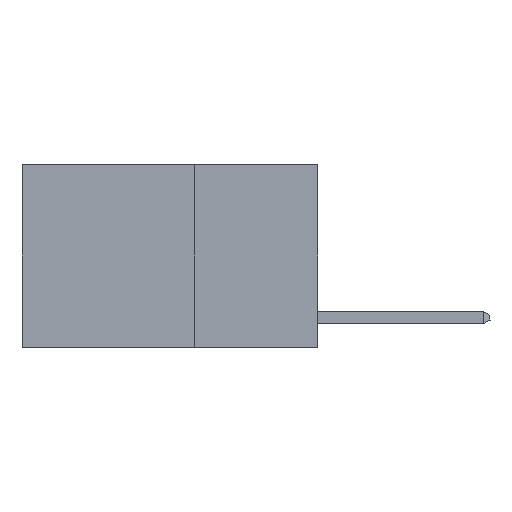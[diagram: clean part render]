
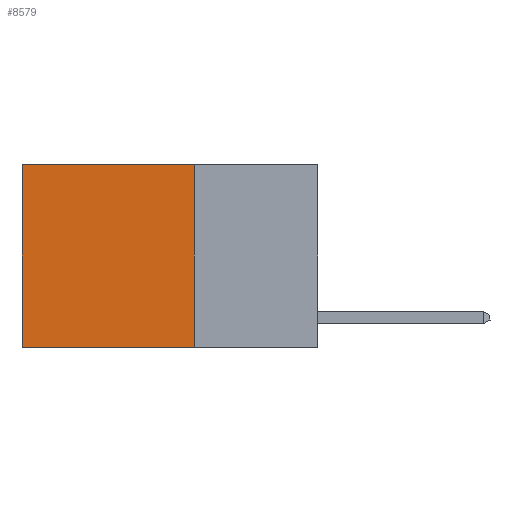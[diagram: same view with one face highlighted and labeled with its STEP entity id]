
A CAD part, left-side view. The second image highlights one B-rep face of the part: STEP entity #8579.
In plain terms, the highlighted planar face has unit normal (-1, 0, 0).
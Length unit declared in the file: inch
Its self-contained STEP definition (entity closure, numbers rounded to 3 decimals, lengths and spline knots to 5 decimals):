
#145 = CARTESIAN_POINT ( 'NONE',  ( 0.2625, 0.25, 0. ) ) ;
#263 = CARTESIAN_POINT ( 'NONE',  ( 0.2625, 0.6, -0.37 ) ) ;
#315 = ORIENTED_EDGE ( 'NONE', *, *, #9654, .F. ) ;
#1732 = VECTOR ( 'NONE', #3383, 39.37008 ) ;
#1985 = VERTEX_POINT ( 'NONE', #4915 ) ;
#2575 = VECTOR ( 'NONE', #4022, 39.37008 ) ;
#3164 = CARTESIAN_POINT ( 'NONE',  ( 0.2625, 0.25, -0.37 ) ) ;
#3243 = CARTESIAN_POINT ( 'NONE',  ( 0.2625, 0.25, 0. ) ) ;
#3383 = DIRECTION ( 'NONE',  ( 0., 0., -1. ) ) ;
#3748 = EDGE_CURVE ( 'NONE', #3813, #4988, #8011, .T. ) ;
#3813 = VERTEX_POINT ( 'NONE', #10590 ) ;
#4022 = DIRECTION ( 'NONE',  ( 0., 0., -1. ) ) ;
#4136 = ORIENTED_EDGE ( 'NONE', *, *, #3748, .T. ) ;
#4202 = FACE_OUTER_BOUND ( 'NONE', #13808, .T. ) ;
#4405 = DIRECTION ( 'NONE',  ( 0., 0., -1. ) ) ;
#4915 = CARTESIAN_POINT ( 'NONE',  ( 0.2625, 0.25, 0. ) ) ;
#4988 = VERTEX_POINT ( 'NONE', #263 ) ;
#5365 = EDGE_CURVE ( 'NONE', #7606, #4988, #7388, .T. ) ;
#7388 = LINE ( 'NONE', #3164, #13209 ) ;
#7606 = VERTEX_POINT ( 'NONE', #14103 ) ;
#7917 = DIRECTION ( 'NONE',  ( 0., 1., 0. ) ) ;
#8011 = LINE ( 'NONE', #15062, #1732 ) ;
#8446 = ORIENTED_EDGE ( 'NONE', *, *, #11267, .T. ) ;
#8579 = ADVANCED_FACE ( 'NONE', ( #4202 ), #10300, .F. ) ;
#9528 = LINE ( 'NONE', #145, #12562 ) ;
#9571 = DIRECTION ( 'NONE',  ( 0., 1., 0. ) ) ;
#9654 = EDGE_CURVE ( 'NONE', #1985, #7606, #11912, .T. ) ;
#10300 = PLANE ( 'NONE',  #13933 ) ;
#10590 = CARTESIAN_POINT ( 'NONE',  ( 0.2625, 0.6, 0. ) ) ;
#11267 = EDGE_CURVE ( 'NONE', #1985, #3813, #9528, .T. ) ;
#11457 = DIRECTION ( 'NONE',  ( 1., 0., 0. ) ) ;
#11912 = LINE ( 'NONE', #12270, #2575 ) ;
#12270 = CARTESIAN_POINT ( 'NONE',  ( 0.2625, 0.25, 0. ) ) ;
#12562 = VECTOR ( 'NONE', #9571, 39.37008 ) ;
#12714 = ORIENTED_EDGE ( 'NONE', *, *, #5365, .F. ) ;
#13209 = VECTOR ( 'NONE', #7917, 39.37008 ) ;
#13808 = EDGE_LOOP ( 'NONE', ( #4136, #12714, #315, #8446 ) ) ;
#13933 = AXIS2_PLACEMENT_3D ( 'NONE', #3243, #11457, #4405 ) ;
#14103 = CARTESIAN_POINT ( 'NONE',  ( 0.2625, 0.25, -0.37 ) ) ;
#15062 = CARTESIAN_POINT ( 'NONE',  ( 0.2625, 0.6, 0. ) ) ;
